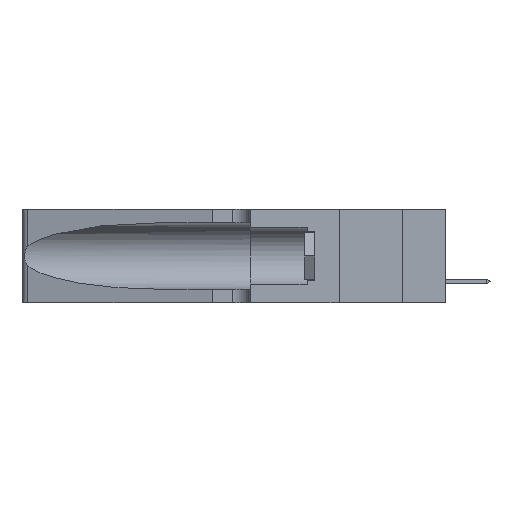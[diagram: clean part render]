
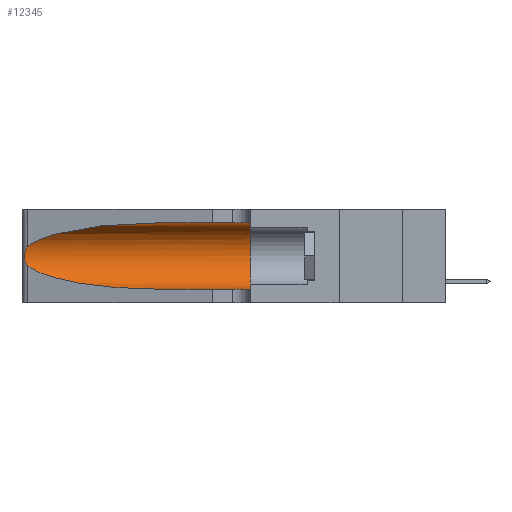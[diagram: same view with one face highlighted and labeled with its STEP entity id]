
A CAD part, left-side view. The second image highlights one B-rep face of the part: STEP entity #12345.
In plain terms, the highlighted cylindrical face has radius 3.308 mm (diameter 6.617 mm), a partial arc.
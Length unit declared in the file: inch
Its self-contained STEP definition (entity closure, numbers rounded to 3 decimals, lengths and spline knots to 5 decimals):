
#977 = CARTESIAN_POINT ( 'NONE',  ( 0.1305, 1.61858, 0.185 ) ) ;
#2210 = CARTESIAN_POINT ( 'NONE',  ( 0.1305, 0.35, 0.31525 ) ) ;
#4154 = CARTESIAN_POINT ( 'NONE',  ( 0.2373, 1.15595, 0.28018 ) ) ;
#4244 = EDGE_CURVE ( 'NONE', #37927, #21214, #36902, .T. ) ;
#4300 = EDGE_CURVE ( 'NONE', #30495, #37927, #16162, .T. ) ;
#4605 = DIRECTION ( 'NONE',  ( 0., 0., -1. ) ) ;
#5541 = AXIS2_PLACEMENT_3D ( 'NONE', #977, #11345, #4605 ) ;
#6058 = FACE_OUTER_BOUND ( 'NONE', #36988, .T. ) ;
#6421 = CARTESIAN_POINT ( 'NONE',  ( 0.18966, 0.96281, 0.05475 ) ) ;
#7327 = CARTESIAN_POINT ( 'NONE',  ( 0.26075, 1.23896, 0.178 ) ) ;
#7744 = CARTESIAN_POINT ( 'NONE',  ( 0.25555, 1.22993, 0.14849 ) ) ;
#8035 = ORIENTED_EDGE ( 'NONE', *, *, #10560, .T. ) ;
#10063 =( BOUNDED_CURVE ( )  B_SPLINE_CURVE ( 3, ( #22270, #38559, #6421, #22657 ),
 .UNSPECIFIED., .F., .T. ) 
 B_SPLINE_CURVE_WITH_KNOTS ( ( 4, 4 ),
 ( 3.44316, 4.71239 ),
 .UNSPECIFIED. ) 
 CURVE ( )  GEOMETRIC_REPRESENTATION_ITEM ( )  RATIONAL_B_SPLINE_CURVE ( ( 1., 0.87, 0.87, 1. ) ) 
 REPRESENTATION_ITEM ( '' )  );
#10172 = VECTOR ( 'NONE', #30232, 39.37008 ) ;
#10560 = EDGE_CURVE ( 'NONE', #30495, #37090, #30875, .T. ) ;
#10561 = CARTESIAN_POINT ( 'NONE',  ( 0.26075, 1.23896, 0.19203 ) ) ;
#10992 = CARTESIAN_POINT ( 'NONE',  ( 0.25789, 1.23486, 0.15765 ) ) ;
#11136 = CARTESIAN_POINT ( 'NONE',  ( 0.25639, 1.23186, 0.15144 ) ) ;
#11345 = DIRECTION ( 'NONE',  ( 0., -1., 0. ) ) ;
#12345 = ADVANCED_FACE ( 'NONE', ( #6058 ), #24641, .F. ) ;
#13514 = ORIENTED_EDGE ( 'NONE', *, *, #20646, .T. ) ;
#13586 = VERTEX_POINT ( 'NONE', #16164 ) ;
#13841 = CARTESIAN_POINT ( 'NONE',  ( 0.25487, 1.22718, 0.22369 ) ) ;
#15135 = CARTESIAN_POINT ( 'NONE',  ( 0.1305, 0.72297, 0.05475 ) ) ;
#15253 = VERTEX_POINT ( 'NONE', #15135 ) ;
#16162 = LINE ( 'NONE', #33058, #10172 ) ;
#16164 = CARTESIAN_POINT ( 'NONE',  ( 0.25487, 1.22718, 0.14631 ) ) ;
#16414 = CARTESIAN_POINT ( 'NONE',  ( 0.26018, 1.23835, 0.19895 ) ) ;
#16705 = CARTESIAN_POINT ( 'NONE',  ( 0.25639, 1.23184, 0.21858 ) ) ;
#17039 = CARTESIAN_POINT ( 'NONE',  ( 0.25487, 1.22718, 0.22369 ) ) ;
#17166 = DIRECTION ( 'NONE',  ( 0., -1., 0. ) ) ;
#18661 = EDGE_CURVE ( 'NONE', #15253, #21214, #38696, .T. ) ;
#18957 = EDGE_CURVE ( 'NONE', #37090, #13586, #29548, .T. ) ;
#20240 = CARTESIAN_POINT ( 'NONE',  ( 0.26017, 1.23833, 0.17102 ) ) ;
#20646 = EDGE_CURVE ( 'NONE', #13586, #15253, #10063, .T. ) ;
#21214 = VERTEX_POINT ( 'NONE', #27658 ) ;
#21758 = VECTOR ( 'NONE', #17166, 39.37008 ) ;
#22270 = CARTESIAN_POINT ( 'NONE',  ( 0.25487, 1.22718, 0.14631 ) ) ;
#22657 = CARTESIAN_POINT ( 'NONE',  ( 0.1305, 0.72297, 0.05475 ) ) ;
#22860 = DIRECTION ( 'NONE',  ( 0., 1., 0. ) ) ;
#23505 = CARTESIAN_POINT ( 'NONE',  ( 0.18966, 0.96281, 0.31525 ) ) ;
#23735 = CARTESIAN_POINT ( 'NONE',  ( 0.25856, 1.23593, 0.16098 ) ) ;
#24366 = ORIENTED_EDGE ( 'NONE', *, *, #4244, .F. ) ;
#24577 = ORIENTED_EDGE ( 'NONE', *, *, #18661, .T. ) ;
#24641 = CYLINDRICAL_SURFACE ( 'NONE', #5541, 0.13025 ) ;
#26126 = ORIENTED_EDGE ( 'NONE', *, *, #4300, .F. ) ;
#26950 = ORIENTED_EDGE ( 'NONE', *, *, #18957, .T. ) ;
#27658 = CARTESIAN_POINT ( 'NONE',  ( 0.1305, 0.35, 0.05475 ) ) ;
#29231 = DIRECTION ( 'NONE',  ( 0., 0., 1. ) ) ;
#29397 = CARTESIAN_POINT ( 'NONE',  ( 0.25487, 1.22718, 0.22369 ) ) ;
#29548 = B_SPLINE_CURVE_WITH_KNOTS ( 'NONE', 3,
 ( #29397, #35832, #16705, #39096, #35565, #16414, #10561, #7327, #20240, #23735, #10992, #11136, #7744, #32943 ),
 .UNSPECIFIED., .F., .F.,
 ( 4, 2, 2, 2, 2, 2, 4 ),
 ( 0., 0.00027, 0.00053, 0.00107, 0.0016, 0.00187, 0.00214 ),
 .UNSPECIFIED. ) ;
#29715 = CARTESIAN_POINT ( 'NONE',  ( 0.1305, 1.61858, 0.05475 ) ) ;
#30232 = DIRECTION ( 'NONE',  ( 0., -1., 0. ) ) ;
#30438 = AXIS2_PLACEMENT_3D ( 'NONE', #35404, #22860, #29231 ) ;
#30495 = VERTEX_POINT ( 'NONE', #31434 ) ;
#30875 =( BOUNDED_CURVE ( )  B_SPLINE_CURVE ( 3, ( #39262, #23505, #4154, #17039 ),
 .UNSPECIFIED., .F., .T. ) 
 B_SPLINE_CURVE_WITH_KNOTS ( ( 4, 4 ),
 ( 1.5708, 2.84003 ),
 .UNSPECIFIED. ) 
 CURVE ( )  GEOMETRIC_REPRESENTATION_ITEM ( )  RATIONAL_B_SPLINE_CURVE ( ( 1., 0.87, 0.87, 1. ) ) 
 REPRESENTATION_ITEM ( '' )  );
#31434 = CARTESIAN_POINT ( 'NONE',  ( 0.1305, 0.72297, 0.31525 ) ) ;
#32943 = CARTESIAN_POINT ( 'NONE',  ( 0.25487, 1.22718, 0.14631 ) ) ;
#33058 = CARTESIAN_POINT ( 'NONE',  ( 0.1305, 1.61858, 0.31525 ) ) ;
#35404 = CARTESIAN_POINT ( 'NONE',  ( 0.1305, 0.35, 0.185 ) ) ;
#35565 = CARTESIAN_POINT ( 'NONE',  ( 0.25854, 1.2359, 0.20912 ) ) ;
#35832 = CARTESIAN_POINT ( 'NONE',  ( 0.25555, 1.22994, 0.2215 ) ) ;
#36902 = CIRCLE ( 'NONE', #30438, 0.13025 ) ;
#36988 = EDGE_LOOP ( 'NONE', ( #8035, #26950, #13514, #24577, #24366, #26126 ) ) ;
#37090 = VERTEX_POINT ( 'NONE', #13841 ) ;
#37927 = VERTEX_POINT ( 'NONE', #2210 ) ;
#38559 = CARTESIAN_POINT ( 'NONE',  ( 0.2373, 1.15595, 0.08982 ) ) ;
#38696 = LINE ( 'NONE', #29715, #21758 ) ;
#39096 = CARTESIAN_POINT ( 'NONE',  ( 0.25787, 1.23484, 0.2124 ) ) ;
#39262 = CARTESIAN_POINT ( 'NONE',  ( 0.1305, 0.72297, 0.31525 ) ) ;
